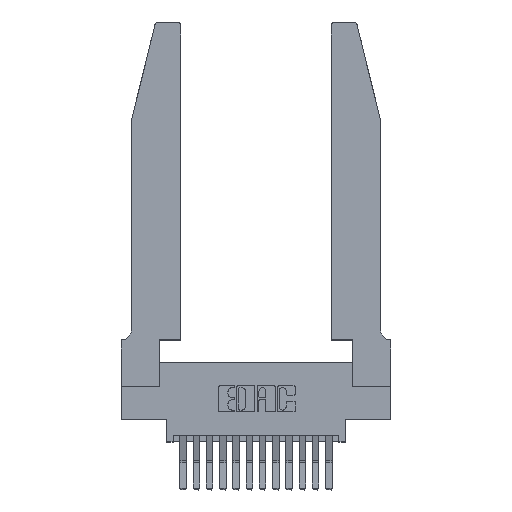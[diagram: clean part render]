
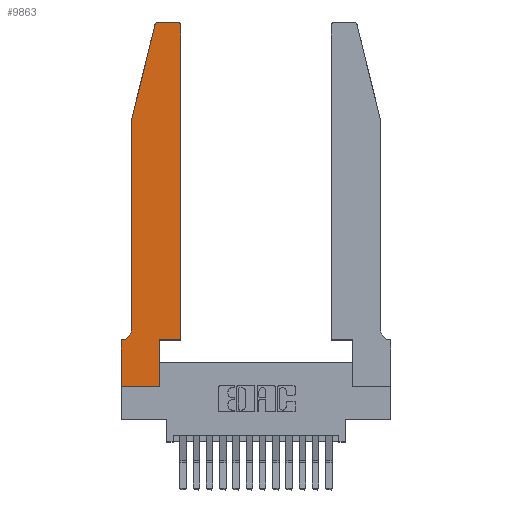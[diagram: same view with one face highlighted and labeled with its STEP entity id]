
A CAD part, top view. The second image highlights one B-rep face of the part: STEP entity #9863.
In plain terms, the highlighted planar face has unit normal (0, 0, 1).
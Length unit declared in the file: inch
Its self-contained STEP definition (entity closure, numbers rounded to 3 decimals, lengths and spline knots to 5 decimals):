
#69 = CARTESIAN_POINT ( 'NONE',  ( 0.0755, 2., 0.37 ) ) ;
#74 = AXIS2_PLACEMENT_3D ( 'NONE', #12326, #15112, #980 ) ;
#99 = DIRECTION ( 'NONE',  ( 0., 1., 0. ) ) ;
#458 = VERTEX_POINT ( 'NONE', #13564 ) ;
#515 = DIRECTION ( 'NONE',  ( -1., 0., 0. ) ) ;
#980 = DIRECTION ( 'NONE',  ( 1., 0., 0. ) ) ;
#1066 = LINE ( 'NONE', #14261, #1479 ) ;
#1102 = CARTESIAN_POINT ( 'NONE',  ( 0.0055, 0.35, 0.37 ) ) ;
#1243 = CIRCLE ( 'NONE', #11375, 0.07 ) ;
#1284 = VERTEX_POINT ( 'NONE', #11288 ) ;
#1289 = EDGE_CURVE ( 'NONE', #3165, #4098, #17641, .T. ) ;
#1479 = VECTOR ( 'NONE', #5536, 39.37008 ) ;
#1510 = EDGE_CURVE ( 'NONE', #6122, #4172, #14059, .T. ) ;
#2134 = VECTOR ( 'NONE', #2171, 39.37008 ) ;
#2171 = DIRECTION ( 'NONE',  ( 1., 0., 0. ) ) ;
#2356 = CARTESIAN_POINT ( 'NONE',  ( 0.25487, 2.72718, 0.37 ) ) ;
#2585 = CARTESIAN_POINT ( 'NONE',  ( 0.0755, 2., 0.37 ) ) ;
#2728 = ORIENTED_EDGE ( 'NONE', *, *, #13762, .T. ) ;
#3086 = EDGE_CURVE ( 'NONE', #14507, #7526, #17993, .T. ) ;
#3098 = CARTESIAN_POINT ( 'NONE',  ( 0.284, 2.72, 0.37 ) ) ;
#3165 = VERTEX_POINT ( 'NONE', #13444 ) ;
#3304 = CIRCLE ( 'NONE', #4441, 0.03 ) ;
#3420 = ORIENTED_EDGE ( 'NONE', *, *, #14647, .T. ) ;
#3822 = DIRECTION ( 'NONE',  ( 1., 0., 0. ) ) ;
#3875 = DIRECTION ( 'NONE',  ( -1., 0., 0. ) ) ;
#3912 = ORIENTED_EDGE ( 'NONE', *, *, #3086, .T. ) ;
#4098 = VERTEX_POINT ( 'NONE', #13663 ) ;
#4172 = VERTEX_POINT ( 'NONE', #5948 ) ;
#4441 = AXIS2_PLACEMENT_3D ( 'NONE', #5051, #10914, #3822 ) ;
#4786 = EDGE_CURVE ( 'NONE', #4098, #9282, #7077, .T. ) ;
#4836 = EDGE_CURVE ( 'NONE', #7526, #5819, #9513, .T. ) ;
#5051 = CARTESIAN_POINT ( 'NONE',  ( 0.4205, 2.72, 0.37 ) ) ;
#5177 = PLANE ( 'NONE',  #74 ) ;
#5212 = VECTOR ( 'NONE', #3875, 39.37008 ) ;
#5360 = CARTESIAN_POINT ( 'NONE',  ( 0.0755, 0.35, 0.37 ) ) ;
#5473 = CARTESIAN_POINT ( 'NONE',  ( 0.284, 2.75, 0.37 ) ) ;
#5536 = DIRECTION ( 'NONE',  ( 0., 1., 0. ) ) ;
#5592 = ORIENTED_EDGE ( 'NONE', *, *, #13938, .T. ) ;
#5819 = VERTEX_POINT ( 'NONE', #2356 ) ;
#5857 = LINE ( 'NONE', #16438, #13420 ) ;
#5948 = CARTESIAN_POINT ( 'NONE',  ( 0.0755, 0.42, 0.37 ) ) ;
#5959 = DIRECTION ( 'NONE',  ( 1., 0., 0. ) ) ;
#6122 = VERTEX_POINT ( 'NONE', #69 ) ;
#6423 = AXIS2_PLACEMENT_3D ( 'NONE', #3098, #13041, #5959 ) ;
#6526 = ORIENTED_EDGE ( 'NONE', *, *, #11363, .T. ) ;
#6532 = VECTOR ( 'NONE', #99, 39.37008 ) ;
#6625 = VERTEX_POINT ( 'NONE', #12647 ) ;
#6973 = EDGE_LOOP ( 'NONE', ( #3912, #17485, #13765, #8137, #3420, #12306, #6526, #9739, #16170, #13207, #5592, #2728 ) ) ;
#7024 = FACE_OUTER_BOUND ( 'NONE', #6973, .T. ) ;
#7077 = LINE ( 'NONE', #11634, #13282 ) ;
#7330 = VECTOR ( 'NONE', #515, 39.37008 ) ;
#7526 = VERTEX_POINT ( 'NONE', #5473 ) ;
#8137 = ORIENTED_EDGE ( 'NONE', *, *, #1510, .T. ) ;
#8600 = CARTESIAN_POINT ( 'NONE',  ( 0.0755, 2., 0.37 ) ) ;
#8872 = DIRECTION ( 'NONE',  ( -1., 0., 0. ) ) ;
#9066 = EDGE_CURVE ( 'NONE', #6625, #3165, #11491, .T. ) ;
#9114 = CARTESIAN_POINT ( 'NONE',  ( 0.2605, 2.75, 0.37 ) ) ;
#9282 = VERTEX_POINT ( 'NONE', #14433 ) ;
#9513 = CIRCLE ( 'NONE', #6423, 0.03 ) ;
#9699 = CARTESIAN_POINT ( 'NONE',  ( 0.4205, 2.75, 0.37 ) ) ;
#9739 = ORIENTED_EDGE ( 'NONE', *, *, #9066, .T. ) ;
#9863 = ADVANCED_FACE ( 'NONE', ( #7024 ), #5177, .T. ) ;
#9878 = EDGE_CURVE ( 'NONE', #17544, #1284, #15218, .T. ) ;
#10291 = VECTOR ( 'NONE', #11243, 39.37008 ) ;
#10607 = DIRECTION ( 'NONE',  ( 0., -1., 0. ) ) ;
#10914 = DIRECTION ( 'NONE',  ( 0., 0., 1. ) ) ;
#11243 = DIRECTION ( 'NONE',  ( -0.239, -0.971, 0. ) ) ;
#11288 = CARTESIAN_POINT ( 'NONE',  ( 0., 0.35, 0.37 ) ) ;
#11363 = EDGE_CURVE ( 'NONE', #1284, #6625, #5857, .T. ) ;
#11375 = AXIS2_PLACEMENT_3D ( 'NONE', #11678, #13217, #8872 ) ;
#11491 = LINE ( 'NONE', #13604, #2134 ) ;
#11634 = CARTESIAN_POINT ( 'NONE',  ( 0.4505, 0.35, 0.37 ) ) ;
#11678 = CARTESIAN_POINT ( 'NONE',  ( 0.0055, 0.42, 0.37 ) ) ;
#12306 = ORIENTED_EDGE ( 'NONE', *, *, #9878, .T. ) ;
#12326 = CARTESIAN_POINT ( 'NONE',  ( 0., 0.35, 0.37 ) ) ;
#12647 = CARTESIAN_POINT ( 'NONE',  ( 0., 0., 0.37 ) ) ;
#12865 = DIRECTION ( 'NONE',  ( 1., 0., 0. ) ) ;
#12882 = CARTESIAN_POINT ( 'NONE',  ( 0.2865, 0.35, 0.37 ) ) ;
#13041 = DIRECTION ( 'NONE',  ( 0., 0., 1. ) ) ;
#13207 = ORIENTED_EDGE ( 'NONE', *, *, #4786, .T. ) ;
#13217 = DIRECTION ( 'NONE',  ( 0., 0., -1. ) ) ;
#13282 = VECTOR ( 'NONE', #12865, 39.37008 ) ;
#13420 = VECTOR ( 'NONE', #10607, 39.37008 ) ;
#13444 = CARTESIAN_POINT ( 'NONE',  ( 0.2865, 0., 0.37 ) ) ;
#13544 = DIRECTION ( 'NONE',  ( 0., -1., 0. ) ) ;
#13564 = CARTESIAN_POINT ( 'NONE',  ( 0.4505, 2.72, 0.37 ) ) ;
#13604 = CARTESIAN_POINT ( 'NONE',  ( 0., 0., 0.37 ) ) ;
#13663 = CARTESIAN_POINT ( 'NONE',  ( 0.2865, 0.35, 0.37 ) ) ;
#13762 = EDGE_CURVE ( 'NONE', #458, #14507, #3304, .T. ) ;
#13765 = ORIENTED_EDGE ( 'NONE', *, *, #15011, .T. ) ;
#13938 = EDGE_CURVE ( 'NONE', #9282, #458, #1066, .T. ) ;
#14059 = LINE ( 'NONE', #8600, #14265 ) ;
#14261 = CARTESIAN_POINT ( 'NONE',  ( 0.4505, 0.35, 0.37 ) ) ;
#14265 = VECTOR ( 'NONE', #13544, 39.37008 ) ;
#14433 = CARTESIAN_POINT ( 'NONE',  ( 0.4505, 0.35, 0.37 ) ) ;
#14507 = VERTEX_POINT ( 'NONE', #9699 ) ;
#14647 = EDGE_CURVE ( 'NONE', #4172, #17544, #1243, .T. ) ;
#15011 = EDGE_CURVE ( 'NONE', #5819, #6122, #17840, .T. ) ;
#15112 = DIRECTION ( 'NONE',  ( 0., 0., 1. ) ) ;
#15218 = LINE ( 'NONE', #5360, #5212 ) ;
#16170 = ORIENTED_EDGE ( 'NONE', *, *, #1289, .T. ) ;
#16438 = CARTESIAN_POINT ( 'NONE',  ( 0., 0., 0.37 ) ) ;
#17485 = ORIENTED_EDGE ( 'NONE', *, *, #4836, .T. ) ;
#17544 = VERTEX_POINT ( 'NONE', #1102 ) ;
#17641 = LINE ( 'NONE', #12882, #6532 ) ;
#17840 = LINE ( 'NONE', #2585, #10291 ) ;
#17993 = LINE ( 'NONE', #9114, #7330 ) ;
